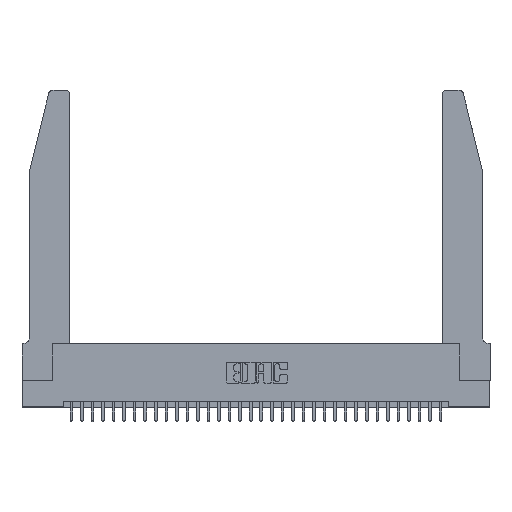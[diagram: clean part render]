
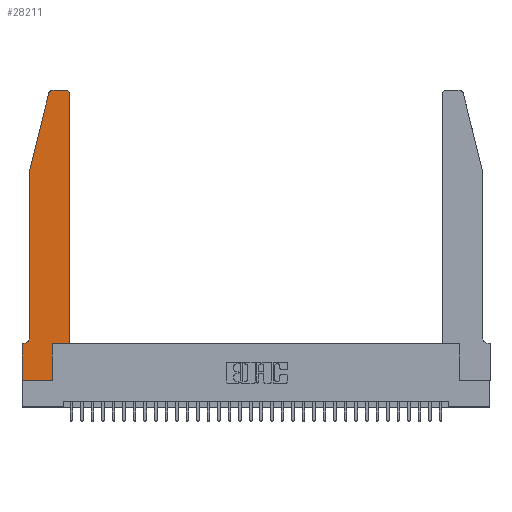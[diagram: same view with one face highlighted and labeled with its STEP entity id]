
A CAD part, top view. The second image highlights one B-rep face of the part: STEP entity #28211.
In plain terms, the highlighted planar face has unit normal (0, 0, 1).
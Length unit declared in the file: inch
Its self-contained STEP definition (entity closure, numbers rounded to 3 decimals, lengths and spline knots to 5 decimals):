
#262 = VERTEX_POINT ( 'NONE', #5155 ) ;
#595 = VERTEX_POINT ( 'NONE', #5442 ) ;
#1187 = AXIS2_PLACEMENT_3D ( 'NONE', #24406, #8689, #27009 ) ;
#1495 = PLANE ( 'NONE',  #7327 ) ;
#1592 = DIRECTION ( 'NONE',  ( 0., 0., 1. ) ) ;
#1841 = CARTESIAN_POINT ( 'NONE',  ( 0.2865, 0.35, 0.37 ) ) ;
#2841 = LINE ( 'NONE', #5779, #16871 ) ;
#2897 = DIRECTION ( 'NONE',  ( 0., 0., -1. ) ) ;
#2975 = ORIENTED_EDGE ( 'NONE', *, *, #24314, .T. ) ;
#3231 = CIRCLE ( 'NONE', #1187, 0.03 ) ;
#3235 = ORIENTED_EDGE ( 'NONE', *, *, #9969, .T. ) ;
#3371 = VECTOR ( 'NONE', #10093, 39.37008 ) ;
#3407 = VERTEX_POINT ( 'NONE', #19227 ) ;
#3505 = VERTEX_POINT ( 'NONE', #22197 ) ;
#3857 = ORIENTED_EDGE ( 'NONE', *, *, #30777, .T. ) ;
#4150 = VERTEX_POINT ( 'NONE', #14459 ) ;
#5146 = VERTEX_POINT ( 'NONE', #15558 ) ;
#5155 = CARTESIAN_POINT ( 'NONE',  ( 0.0055, 0.35, 0.37 ) ) ;
#5442 = CARTESIAN_POINT ( 'NONE',  ( 0.2865, 0.35, 0.37 ) ) ;
#5767 = VERTEX_POINT ( 'NONE', #15185 ) ;
#5779 = CARTESIAN_POINT ( 'NONE',  ( 0.0755, 0.35, 0.37 ) ) ;
#5954 = ORIENTED_EDGE ( 'NONE', *, *, #15816, .T. ) ;
#6129 = LINE ( 'NONE', #25353, #26250 ) ;
#6357 = ORIENTED_EDGE ( 'NONE', *, *, #23463, .T. ) ;
#6372 = DIRECTION ( 'NONE',  ( 1., 0., 0. ) ) ;
#6790 = DIRECTION ( 'NONE',  ( 0., 0., 1. ) ) ;
#6838 = VECTOR ( 'NONE', #20166, 39.37008 ) ;
#6961 = DIRECTION ( 'NONE',  ( 1., 0., 0. ) ) ;
#7327 = AXIS2_PLACEMENT_3D ( 'NONE', #17283, #6790, #25172 ) ;
#8165 = EDGE_CURVE ( 'NONE', #595, #20541, #8739, .T. ) ;
#8689 = DIRECTION ( 'NONE',  ( 0., 0., 1. ) ) ;
#8739 = LINE ( 'NONE', #22154, #21916 ) ;
#8830 = EDGE_CURVE ( 'NONE', #24027, #22360, #29963, .T. ) ;
#9011 = ORIENTED_EDGE ( 'NONE', *, *, #31419, .T. ) ;
#9412 = CARTESIAN_POINT ( 'NONE',  ( 0.0755, 0.42, 0.37 ) ) ;
#9626 = EDGE_CURVE ( 'NONE', #3505, #5767, #6129, .T. ) ;
#9789 = ORIENTED_EDGE ( 'NONE', *, *, #13958, .T. ) ;
#9969 = EDGE_CURVE ( 'NONE', #5146, #29690, #3231, .T. ) ;
#10093 = DIRECTION ( 'NONE',  ( 0., 1., 0. ) ) ;
#12600 = VECTOR ( 'NONE', #14984, 39.37008 ) ;
#12723 = VECTOR ( 'NONE', #22890, 39.37008 ) ;
#13374 = ORIENTED_EDGE ( 'NONE', *, *, #9626, .T. ) ;
#13958 = EDGE_CURVE ( 'NONE', #5767, #595, #15214, .T. ) ;
#14459 = CARTESIAN_POINT ( 'NONE',  ( 0.284, 2.75, 0.37 ) ) ;
#14962 = AXIS2_PLACEMENT_3D ( 'NONE', #18682, #2897, #21339 ) ;
#14984 = DIRECTION ( 'NONE',  ( 0., -1., 0. ) ) ;
#15184 = CARTESIAN_POINT ( 'NONE',  ( 0.2605, 2.75, 0.37 ) ) ;
#15185 = CARTESIAN_POINT ( 'NONE',  ( 0.2865, 0., 0.37 ) ) ;
#15214 = LINE ( 'NONE', #1841, #12723 ) ;
#15324 = EDGE_CURVE ( 'NONE', #30559, #262, #32582, .T. ) ;
#15558 = CARTESIAN_POINT ( 'NONE',  ( 0.4505, 2.72, 0.37 ) ) ;
#15816 = EDGE_CURVE ( 'NONE', #3407, #3505, #26517, .T. ) ;
#16871 = VECTOR ( 'NONE', #26770, 39.37008 ) ;
#17283 = CARTESIAN_POINT ( 'NONE',  ( 0., 0.35, 0.37 ) ) ;
#17394 = CARTESIAN_POINT ( 'NONE',  ( 0.284, 2.72, 0.37 ) ) ;
#17453 = ORIENTED_EDGE ( 'NONE', *, *, #8830, .T. ) ;
#17527 = CARTESIAN_POINT ( 'NONE',  ( 0.0755, 2., 0.37 ) ) ;
#17854 = DIRECTION ( 'NONE',  ( -1., 0., 0. ) ) ;
#18299 = CARTESIAN_POINT ( 'NONE',  ( 0.4505, 0.35, 0.37 ) ) ;
#18303 = ORIENTED_EDGE ( 'NONE', *, *, #15324, .T. ) ;
#18682 = CARTESIAN_POINT ( 'NONE',  ( 0.0055, 0.42, 0.37 ) ) ;
#19227 = CARTESIAN_POINT ( 'NONE',  ( 0., 0.35, 0.37 ) ) ;
#19696 = CIRCLE ( 'NONE', #33253, 0.03 ) ;
#20042 = DIRECTION ( 'NONE',  ( 1., 0., 0. ) ) ;
#20166 = DIRECTION ( 'NONE',  ( 0., -1., 0. ) ) ;
#20541 = VERTEX_POINT ( 'NONE', #18299 ) ;
#21339 = DIRECTION ( 'NONE',  ( -1., 0., 0. ) ) ;
#21681 = LINE ( 'NONE', #17527, #6838 ) ;
#21916 = VECTOR ( 'NONE', #6372, 39.37008 ) ;
#22154 = CARTESIAN_POINT ( 'NONE',  ( 0.4505, 0.35, 0.37 ) ) ;
#22197 = CARTESIAN_POINT ( 'NONE',  ( 0., 0., 0.37 ) ) ;
#22360 = VERTEX_POINT ( 'NONE', #29905 ) ;
#22890 = DIRECTION ( 'NONE',  ( 0., 1., 0. ) ) ;
#23463 = EDGE_CURVE ( 'NONE', #262, #3407, #2841, .T. ) ;
#23576 = CARTESIAN_POINT ( 'NONE',  ( 0.25487, 2.72718, 0.37 ) ) ;
#23879 = VECTOR ( 'NONE', #32249, 39.37008 ) ;
#24027 = VERTEX_POINT ( 'NONE', #23576 ) ;
#24314 = EDGE_CURVE ( 'NONE', #4150, #24027, #19696, .T. ) ;
#24364 = ORIENTED_EDGE ( 'NONE', *, *, #24445, .T. ) ;
#24406 = CARTESIAN_POINT ( 'NONE',  ( 0.4205, 2.72, 0.37 ) ) ;
#24445 = EDGE_CURVE ( 'NONE', #29690, #4150, #31037, .T. ) ;
#24483 = CARTESIAN_POINT ( 'NONE',  ( 0.0755, 2., 0.37 ) ) ;
#25171 = LINE ( 'NONE', #25805, #3371 ) ;
#25172 = DIRECTION ( 'NONE',  ( 1., 0., 0. ) ) ;
#25353 = CARTESIAN_POINT ( 'NONE',  ( 0., 0., 0.37 ) ) ;
#25620 = CARTESIAN_POINT ( 'NONE',  ( 0., 0., 0.37 ) ) ;
#25805 = CARTESIAN_POINT ( 'NONE',  ( 0.4505, 0.35, 0.37 ) ) ;
#26250 = VECTOR ( 'NONE', #6961, 39.37008 ) ;
#26303 = CARTESIAN_POINT ( 'NONE',  ( 0.4205, 2.75, 0.37 ) ) ;
#26517 = LINE ( 'NONE', #25620, #12600 ) ;
#26770 = DIRECTION ( 'NONE',  ( -1., 0., 0. ) ) ;
#27009 = DIRECTION ( 'NONE',  ( 1., 0., 0. ) ) ;
#28211 = ADVANCED_FACE ( 'NONE', ( #30754 ), #1495, .T. ) ;
#29427 = VECTOR ( 'NONE', #17854, 39.37008 ) ;
#29452 = ORIENTED_EDGE ( 'NONE', *, *, #8165, .T. ) ;
#29690 = VERTEX_POINT ( 'NONE', #26303 ) ;
#29905 = CARTESIAN_POINT ( 'NONE',  ( 0.0755, 2., 0.37 ) ) ;
#29963 = LINE ( 'NONE', #24483, #23879 ) ;
#30559 = VERTEX_POINT ( 'NONE', #9412 ) ;
#30754 = FACE_OUTER_BOUND ( 'NONE', #33323, .T. ) ;
#30777 = EDGE_CURVE ( 'NONE', #22360, #30559, #21681, .T. ) ;
#31037 = LINE ( 'NONE', #15184, #29427 ) ;
#31419 = EDGE_CURVE ( 'NONE', #20541, #5146, #25171, .T. ) ;
#32249 = DIRECTION ( 'NONE',  ( -0.239, -0.971, 0. ) ) ;
#32582 = CIRCLE ( 'NONE', #14962, 0.07 ) ;
#33253 = AXIS2_PLACEMENT_3D ( 'NONE', #17394, #1592, #20042 ) ;
#33323 = EDGE_LOOP ( 'NONE', ( #24364, #2975, #17453, #3857, #18303, #6357, #5954, #13374, #9789, #29452, #9011, #3235 ) ) ;
